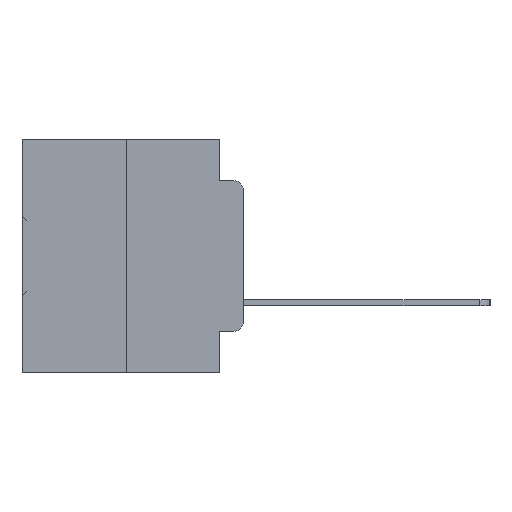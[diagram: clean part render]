
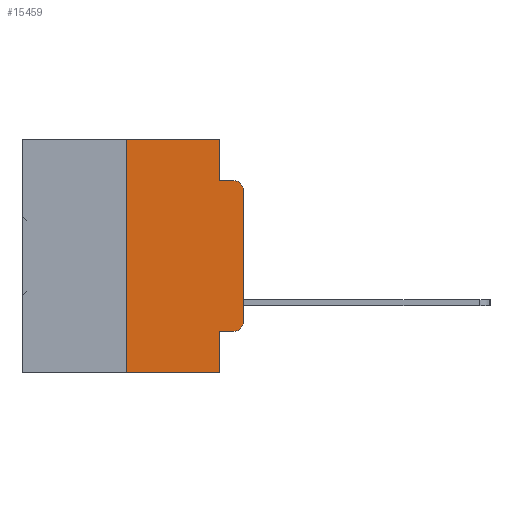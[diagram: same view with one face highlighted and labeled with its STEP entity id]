
A CAD part, left-side view. The second image highlights one B-rep face of the part: STEP entity #15459.
In plain terms, the highlighted planar face has unit normal (-1, 0, 0).
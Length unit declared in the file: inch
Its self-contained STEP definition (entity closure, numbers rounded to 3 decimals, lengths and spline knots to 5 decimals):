
#541 = AXIS2_PLACEMENT_3D ( 'NONE', #18710, #1804, #21494 ) ;
#1370 = VECTOR ( 'NONE', #17382, 39.37008 ) ;
#1804 = DIRECTION ( 'NONE',  ( -1., 0., 0. ) ) ;
#1963 = DIRECTION ( 'NONE',  ( 0., -1., 0. ) ) ;
#2638 = ORIENTED_EDGE ( 'NONE', *, *, #33807, .T. ) ;
#3059 = CARTESIAN_POINT ( 'NONE',  ( 0., 0.051, -0.0885 ) ) ;
#3393 = LINE ( 'NONE', #14635, #17505 ) ;
#3731 = CARTESIAN_POINT ( 'NONE',  ( 0., 0.02, -0.1085 ) ) ;
#4649 = VECTOR ( 'NONE', #14319, 39.37008 ) ;
#5293 = ORIENTED_EDGE ( 'NONE', *, *, #22791, .F. ) ;
#5870 = EDGE_CURVE ( 'NONE', #21082, #29755, #26339, .T. ) ;
#6439 = LINE ( 'NONE', #33397, #4649 ) ;
#6455 = CARTESIAN_POINT ( 'NONE',  ( 0., 0.051, 0. ) ) ;
#6578 = DIRECTION ( 'NONE',  ( 0., 0., -1. ) ) ;
#7823 = EDGE_CURVE ( 'NONE', #9425, #21082, #34454, .T. ) ;
#9054 = AXIS2_PLACEMENT_3D ( 'NONE', #3731, #23338, #6578 ) ;
#9425 = VERTEX_POINT ( 'NONE', #26600 ) ;
#9473 = CARTESIAN_POINT ( 'NONE',  ( 0., 0.473, 0. ) ) ;
#9798 = CARTESIAN_POINT ( 'NONE',  ( 0., 0.051, -0.0885 ) ) ;
#10459 = VERTEX_POINT ( 'NONE', #19946 ) ;
#10779 = VERTEX_POINT ( 'NONE', #35400 ) ;
#11115 = ORIENTED_EDGE ( 'NONE', *, *, #26454, .F. ) ;
#11438 = VERTEX_POINT ( 'NONE', #3059 ) ;
#12328 = PLANE ( 'NONE',  #26376 ) ;
#13303 = LINE ( 'NONE', #14744, #26206 ) ;
#14319 = DIRECTION ( 'NONE',  ( 0., 0., 1. ) ) ;
#14635 = CARTESIAN_POINT ( 'NONE',  ( 0., 0.473, 0. ) ) ;
#14744 = CARTESIAN_POINT ( 'NONE',  ( 0., 0.051, 0. ) ) ;
#15422 = EDGE_CURVE ( 'NONE', #9425, #32730, #21878, .T. ) ;
#15459 = ADVANCED_FACE ( 'NONE', ( #29144 ), #12328, .F. ) ;
#15956 = EDGE_CURVE ( 'NONE', #19638, #27502, #3393, .T. ) ;
#15983 = CARTESIAN_POINT ( 'NONE',  ( 0., 0.473, -0.5 ) ) ;
#16229 = LINE ( 'NONE', #15983, #21838 ) ;
#17227 = ORIENTED_EDGE ( 'NONE', *, *, #15422, .F. ) ;
#17382 = DIRECTION ( 'NONE',  ( 0., 0., 1. ) ) ;
#17392 = DIRECTION ( 'NONE',  ( 0., -1., 0. ) ) ;
#17493 = DIRECTION ( 'NONE',  ( 0., 0., -1. ) ) ;
#17505 = VECTOR ( 'NONE', #17392, 39.37008 ) ;
#17904 = DIRECTION ( 'NONE',  ( 0., 0., -1. ) ) ;
#18645 = CARTESIAN_POINT ( 'NONE',  ( 0., 0.051, -0.5 ) ) ;
#18710 = CARTESIAN_POINT ( 'NONE',  ( 0., 0.02, -0.3915 ) ) ;
#18949 = DIRECTION ( 'NONE',  ( 0., -1., 0. ) ) ;
#18978 = ORIENTED_EDGE ( 'NONE', *, *, #7823, .T. ) ;
#19112 = EDGE_CURVE ( 'NONE', #10459, #19638, #6439, .T. ) ;
#19638 = VERTEX_POINT ( 'NONE', #24848 ) ;
#19946 = CARTESIAN_POINT ( 'NONE',  ( 0., 0.25, -0.5 ) ) ;
#20369 = CIRCLE ( 'NONE', #9054, 0.02 ) ;
#21082 = VERTEX_POINT ( 'NONE', #30642 ) ;
#21494 = DIRECTION ( 'NONE',  ( 0., 0., -1. ) ) ;
#21513 = VECTOR ( 'NONE', #34667, 39.37008 ) ;
#21838 = VECTOR ( 'NONE', #1963, 39.37008 ) ;
#21878 = LINE ( 'NONE', #6455, #35585 ) ;
#22791 = EDGE_CURVE ( 'NONE', #27502, #11438, #13303, .T. ) ;
#22843 = ORIENTED_EDGE ( 'NONE', *, *, #28560, .T. ) ;
#23237 = LINE ( 'NONE', #9798, #21513 ) ;
#23287 = VERTEX_POINT ( 'NONE', #35947 ) ;
#23338 = DIRECTION ( 'NONE',  ( -1., 0., 0. ) ) ;
#23794 = LINE ( 'NONE', #31044, #1370 ) ;
#24848 = CARTESIAN_POINT ( 'NONE',  ( 0., 0.25, 0. ) ) ;
#24958 = ORIENTED_EDGE ( 'NONE', *, *, #30127, .T. ) ;
#26206 = VECTOR ( 'NONE', #17493, 39.37008 ) ;
#26260 = ORIENTED_EDGE ( 'NONE', *, *, #5870, .T. ) ;
#26339 = CIRCLE ( 'NONE', #541, 0.02 ) ;
#26376 = AXIS2_PLACEMENT_3D ( 'NONE', #9473, #34347, #17904 ) ;
#26454 = EDGE_CURVE ( 'NONE', #11438, #10779, #23237, .T. ) ;
#26600 = CARTESIAN_POINT ( 'NONE',  ( 0., 0.051, -0.4115 ) ) ;
#27167 = VECTOR ( 'NONE', #18949, 39.37008 ) ;
#27502 = VERTEX_POINT ( 'NONE', #30854 ) ;
#28560 = EDGE_CURVE ( 'NONE', #10459, #32730, #16229, .T. ) ;
#28704 = DIRECTION ( 'NONE',  ( 0., 0., -1. ) ) ;
#29144 = FACE_OUTER_BOUND ( 'NONE', #31551, .T. ) ;
#29755 = VERTEX_POINT ( 'NONE', #35087 ) ;
#30127 = EDGE_CURVE ( 'NONE', #23287, #10779, #20369, .T. ) ;
#30642 = CARTESIAN_POINT ( 'NONE',  ( 0., 0.02, -0.4115 ) ) ;
#30854 = CARTESIAN_POINT ( 'NONE',  ( 0., 0.051, 0. ) ) ;
#31044 = CARTESIAN_POINT ( 'NONE',  ( 0., 0., 0. ) ) ;
#31551 = EDGE_LOOP ( 'NONE', ( #2638, #24958, #11115, #5293, #34821, #35697, #22843, #17227, #18978, #26260 ) ) ;
#32730 = VERTEX_POINT ( 'NONE', #18645 ) ;
#33397 = CARTESIAN_POINT ( 'NONE',  ( 0., 0.25, 0. ) ) ;
#33807 = EDGE_CURVE ( 'NONE', #29755, #23287, #23794, .T. ) ;
#34347 = DIRECTION ( 'NONE',  ( 1., 0., 0. ) ) ;
#34454 = LINE ( 'NONE', #35371, #27167 ) ;
#34667 = DIRECTION ( 'NONE',  ( 0., -1., 0. ) ) ;
#34821 = ORIENTED_EDGE ( 'NONE', *, *, #15956, .F. ) ;
#35087 = CARTESIAN_POINT ( 'NONE',  ( 0., 0., -0.3915 ) ) ;
#35371 = CARTESIAN_POINT ( 'NONE',  ( 0., 0.051, -0.4115 ) ) ;
#35400 = CARTESIAN_POINT ( 'NONE',  ( 0., 0.02, -0.0885 ) ) ;
#35585 = VECTOR ( 'NONE', #28704, 39.37008 ) ;
#35697 = ORIENTED_EDGE ( 'NONE', *, *, #19112, .F. ) ;
#35947 = CARTESIAN_POINT ( 'NONE',  ( 0., 0., -0.1085 ) ) ;
